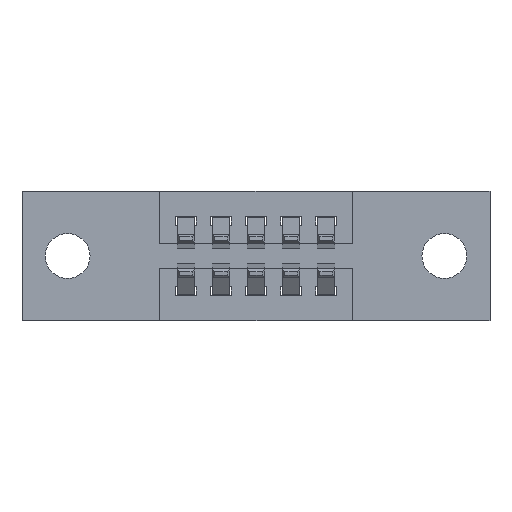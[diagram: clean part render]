
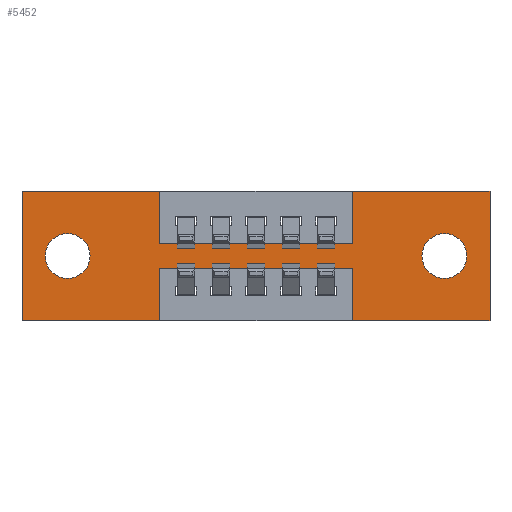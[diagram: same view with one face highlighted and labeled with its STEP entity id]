
A CAD part, front view. The second image highlights one B-rep face of the part: STEP entity #5452.
In plain terms, the highlighted planar face has unit normal (0, -1, 0).
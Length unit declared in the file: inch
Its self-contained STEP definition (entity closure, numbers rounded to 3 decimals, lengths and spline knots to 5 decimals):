
#2 = DIRECTION ( 'NONE',  ( 0., 0., -1. ) ) ;
#36 = DIRECTION ( 'NONE',  ( 0., 0., -1. ) ) ;
#39 = EDGE_CURVE ( 'NONE', #3621, #6244, #7031, .T. ) ;
#106 = DIRECTION ( 'NONE',  ( 0., 1., 0. ) ) ;
#252 = VERTEX_POINT ( 'NONE', #847 ) ;
#265 = EDGE_CURVE ( 'NONE', #8048, #544, #295, .T. ) ;
#295 = CIRCLE ( 'NONE', #8822, 0.064 ) ;
#373 = CARTESIAN_POINT ( 'NONE',  ( 0.13, 0., -0.185 ) ) ;
#383 = EDGE_CURVE ( 'NONE', #5993, #5320, #2974, .T. ) ;
#424 = CARTESIAN_POINT ( 'NONE',  ( 0., 0., -0.37 ) ) ;
#465 = EDGE_CURVE ( 'NONE', #5697, #3621, #6914, .T. ) ;
#513 = VERTEX_POINT ( 'NONE', #7424 ) ;
#544 = VERTEX_POINT ( 'NONE', #3466 ) ;
#576 = CIRCLE ( 'NONE', #2334, 0.064 ) ;
#595 = AXIS2_PLACEMENT_3D ( 'NONE', #7594, #4784, #641 ) ;
#641 = DIRECTION ( 'NONE',  ( 0., 0., -1. ) ) ;
#814 = CARTESIAN_POINT ( 'NONE',  ( 0., 0., 0. ) ) ;
#847 = CARTESIAN_POINT ( 'NONE',  ( 0.13, 0., -0.121 ) ) ;
#896 = VECTOR ( 'NONE', #7299, 39.37008 ) ;
#1010 = VERTEX_POINT ( 'NONE', #7337 ) ;
#1085 = VECTOR ( 'NONE', #2703, 39.37008 ) ;
#1205 = VERTEX_POINT ( 'NONE', #1532 ) ;
#1412 = CARTESIAN_POINT ( 'NONE',  ( 0., 0., 0. ) ) ;
#1504 = FACE_OUTER_BOUND ( 'NONE', #6736, .T. ) ;
#1532 = CARTESIAN_POINT ( 'NONE',  ( 1.335, 0., -0.37 ) ) ;
#1619 = FACE_BOUND ( 'NONE', #7298, .T. ) ;
#1672 = DIRECTION ( 'NONE',  ( 0., 0., -1. ) ) ;
#1675 = ORIENTED_EDGE ( 'NONE', *, *, #5478, .F. ) ;
#1692 = DIRECTION ( 'NONE',  ( 0., 0., 1. ) ) ;
#1828 = LINE ( 'NONE', #4115, #6940 ) ;
#2002 = ORIENTED_EDGE ( 'NONE', *, *, #7427, .F. ) ;
#2042 = ORIENTED_EDGE ( 'NONE', *, *, #8536, .F. ) ;
#2061 = CARTESIAN_POINT ( 'NONE',  ( 0.3925, 0., -0.37 ) ) ;
#2174 = LINE ( 'NONE', #6180, #1085 ) ;
#2257 = CARTESIAN_POINT ( 'NONE',  ( 1.205, 0., -0.249 ) ) ;
#2334 = AXIS2_PLACEMENT_3D ( 'NONE', #6567, #4472, #6598 ) ;
#2370 = VERTEX_POINT ( 'NONE', #8610 ) ;
#2431 = CARTESIAN_POINT ( 'NONE',  ( 0.9425, 0., -0.37 ) ) ;
#2541 = CARTESIAN_POINT ( 'NONE',  ( 0.9425, 0., 0. ) ) ;
#2675 = ORIENTED_EDGE ( 'NONE', *, *, #7902, .F. ) ;
#2697 = CARTESIAN_POINT ( 'NONE',  ( 0.3925, 0., -0.22 ) ) ;
#2703 = DIRECTION ( 'NONE',  ( -1., 0., 0. ) ) ;
#2761 = CARTESIAN_POINT ( 'NONE',  ( 0.3925, 0., 0. ) ) ;
#2785 = DIRECTION ( 'NONE',  ( 0., 0., 1. ) ) ;
#2855 = EDGE_CURVE ( 'NONE', #5347, #513, #8718, .T. ) ;
#2974 = LINE ( 'NONE', #5167, #5615 ) ;
#3202 = EDGE_LOOP ( 'NONE', ( #7701, #7699 ) ) ;
#3224 = CARTESIAN_POINT ( 'NONE',  ( 0.13, 0., -0.185 ) ) ;
#3254 = LINE ( 'NONE', #2697, #896 ) ;
#3268 = CARTESIAN_POINT ( 'NONE',  ( 0., 0., 0. ) ) ;
#3387 = CARTESIAN_POINT ( 'NONE',  ( 0.3925, 0., -0.22 ) ) ;
#3461 = CARTESIAN_POINT ( 'NONE',  ( 0.9425, 0., -0.15 ) ) ;
#3466 = CARTESIAN_POINT ( 'NONE',  ( 1.205, 0., -0.121 ) ) ;
#3549 = LINE ( 'NONE', #2061, #4593 ) ;
#3560 = VERTEX_POINT ( 'NONE', #7260 ) ;
#3621 = VERTEX_POINT ( 'NONE', #424 ) ;
#4111 = CARTESIAN_POINT ( 'NONE',  ( 0., 0., 0. ) ) ;
#4115 = CARTESIAN_POINT ( 'NONE',  ( 1.335, 0., 0. ) ) ;
#4222 = VECTOR ( 'NONE', #4819, 39.37008 ) ;
#4310 = DIRECTION ( 'NONE',  ( 1., 0., 0. ) ) ;
#4330 = VECTOR ( 'NONE', #4310, 39.37008 ) ;
#4472 = DIRECTION ( 'NONE',  ( 0., 1., 0. ) ) ;
#4543 = CARTESIAN_POINT ( 'NONE',  ( 0., 0., -0.37 ) ) ;
#4554 = VECTOR ( 'NONE', #1672, 39.37008 ) ;
#4589 = CARTESIAN_POINT ( 'NONE',  ( 0.9425, 0., -0.37 ) ) ;
#4593 = VECTOR ( 'NONE', #36, 39.37008 ) ;
#4659 = EDGE_CURVE ( 'NONE', #2370, #5993, #7606, .T. ) ;
#4784 = DIRECTION ( 'NONE',  ( 0., -1., 0. ) ) ;
#4819 = DIRECTION ( 'NONE',  ( 1., 0., 0. ) ) ;
#4842 = VECTOR ( 'NONE', #7387, 39.37008 ) ;
#4928 = EDGE_CURVE ( 'NONE', #1205, #5347, #2174, .T. ) ;
#5062 = CARTESIAN_POINT ( 'NONE',  ( 0.3925, 0., -0.15 ) ) ;
#5124 = ORIENTED_EDGE ( 'NONE', *, *, #465, .F. ) ;
#5146 = CARTESIAN_POINT ( 'NONE',  ( 0.3925, 0., 0. ) ) ;
#5167 = CARTESIAN_POINT ( 'NONE',  ( 0.9425, 0., 0. ) ) ;
#5278 = AXIS2_PLACEMENT_3D ( 'NONE', #3224, #5967, #6790 ) ;
#5320 = VERTEX_POINT ( 'NONE', #2541 ) ;
#5347 = VERTEX_POINT ( 'NONE', #4589 ) ;
#5452 = ADVANCED_FACE ( 'NONE', ( #1619, #8575, #1504 ), #6892, .T. ) ;
#5478 = EDGE_CURVE ( 'NONE', #1010, #1205, #1828, .T. ) ;
#5500 = ORIENTED_EDGE ( 'NONE', *, *, #265, .T. ) ;
#5615 = VECTOR ( 'NONE', #1692, 39.37008 ) ;
#5683 = EDGE_CURVE ( 'NONE', #8134, #5697, #3549, .T. ) ;
#5697 = VERTEX_POINT ( 'NONE', #8247 ) ;
#5718 = VERTEX_POINT ( 'NONE', #2761 ) ;
#5779 = AXIS2_PLACEMENT_3D ( 'NONE', #373, #106, #7285 ) ;
#5956 = DIRECTION ( 'NONE',  ( 0., 0., 1. ) ) ;
#5967 = DIRECTION ( 'NONE',  ( 0., 1., 0. ) ) ;
#5979 = EDGE_CURVE ( 'NONE', #252, #3560, #7873, .T. ) ;
#5980 = DIRECTION ( 'NONE',  ( 1., 0., 0. ) ) ;
#5993 = VERTEX_POINT ( 'NONE', #3461 ) ;
#6180 = CARTESIAN_POINT ( 'NONE',  ( 0., 0., -0.37 ) ) ;
#6244 = VERTEX_POINT ( 'NONE', #814 ) ;
#6410 = LINE ( 'NONE', #5146, #4554 ) ;
#6411 = CARTESIAN_POINT ( 'NONE',  ( 1.205, 0., -0.185 ) ) ;
#6447 = DIRECTION ( 'NONE',  ( 0., 1., 0. ) ) ;
#6567 = CARTESIAN_POINT ( 'NONE',  ( 1.205, 0., -0.185 ) ) ;
#6598 = DIRECTION ( 'NONE',  ( 0., 0., -1. ) ) ;
#6681 = ORIENTED_EDGE ( 'NONE', *, *, #4659, .F. ) ;
#6688 = ORIENTED_EDGE ( 'NONE', *, *, #5683, .F. ) ;
#6692 = ORIENTED_EDGE ( 'NONE', *, *, #8971, .F. ) ;
#6736 = EDGE_LOOP ( 'NONE', ( #6688, #2002, #7102, #7446, #1675, #6692, #8316, #6681, #2675, #2042, #7879, #5124 ) ) ;
#6790 = DIRECTION ( 'NONE',  ( 0., 0., 1. ) ) ;
#6892 = PLANE ( 'NONE',  #595 ) ;
#6914 = LINE ( 'NONE', #4543, #4842 ) ;
#6940 = VECTOR ( 'NONE', #2, 39.37008 ) ;
#7031 = LINE ( 'NONE', #1412, #7345 ) ;
#7063 = LINE ( 'NONE', #3268, #8706 ) ;
#7075 = VECTOR ( 'NONE', #5956, 39.37008 ) ;
#7102 = ORIENTED_EDGE ( 'NONE', *, *, #2855, .F. ) ;
#7147 = EDGE_CURVE ( 'NONE', #544, #8048, #576, .T. ) ;
#7151 = DIRECTION ( 'NONE',  ( 0., 0., -1. ) ) ;
#7260 = CARTESIAN_POINT ( 'NONE',  ( 0.13, 0., -0.249 ) ) ;
#7285 = DIRECTION ( 'NONE',  ( 0., 0., 1. ) ) ;
#7298 = EDGE_LOOP ( 'NONE', ( #8998, #5500 ) ) ;
#7299 = DIRECTION ( 'NONE',  ( -1., 0., 0. ) ) ;
#7337 = CARTESIAN_POINT ( 'NONE',  ( 1.335, 0., 0. ) ) ;
#7345 = VECTOR ( 'NONE', #2785, 39.37008 ) ;
#7387 = DIRECTION ( 'NONE',  ( -1., 0., 0. ) ) ;
#7424 = CARTESIAN_POINT ( 'NONE',  ( 0.9425, 0., -0.22 ) ) ;
#7427 = EDGE_CURVE ( 'NONE', #513, #8134, #3254, .T. ) ;
#7446 = ORIENTED_EDGE ( 'NONE', *, *, #4928, .F. ) ;
#7571 = EDGE_CURVE ( 'NONE', #3560, #252, #7947, .T. ) ;
#7594 = CARTESIAN_POINT ( 'NONE',  ( 0., 0., -0.37 ) ) ;
#7606 = LINE ( 'NONE', #5062, #4330 ) ;
#7699 = ORIENTED_EDGE ( 'NONE', *, *, #7571, .T. ) ;
#7701 = ORIENTED_EDGE ( 'NONE', *, *, #5979, .T. ) ;
#7710 = LINE ( 'NONE', #4111, #4222 ) ;
#7873 = CIRCLE ( 'NONE', #5779, 0.064 ) ;
#7879 = ORIENTED_EDGE ( 'NONE', *, *, #39, .F. ) ;
#7902 = EDGE_CURVE ( 'NONE', #5718, #2370, #6410, .T. ) ;
#7947 = CIRCLE ( 'NONE', #5278, 0.064 ) ;
#8048 = VERTEX_POINT ( 'NONE', #2257 ) ;
#8134 = VERTEX_POINT ( 'NONE', #3387 ) ;
#8247 = CARTESIAN_POINT ( 'NONE',  ( 0.3925, 0., -0.37 ) ) ;
#8316 = ORIENTED_EDGE ( 'NONE', *, *, #383, .F. ) ;
#8536 = EDGE_CURVE ( 'NONE', #6244, #5718, #7063, .T. ) ;
#8575 = FACE_BOUND ( 'NONE', #3202, .T. ) ;
#8610 = CARTESIAN_POINT ( 'NONE',  ( 0.3925, 0., -0.15 ) ) ;
#8706 = VECTOR ( 'NONE', #5980, 39.37008 ) ;
#8718 = LINE ( 'NONE', #2431, #7075 ) ;
#8822 = AXIS2_PLACEMENT_3D ( 'NONE', #6411, #6447, #7151 ) ;
#8971 = EDGE_CURVE ( 'NONE', #5320, #1010, #7710, .T. ) ;
#8998 = ORIENTED_EDGE ( 'NONE', *, *, #7147, .T. ) ;
